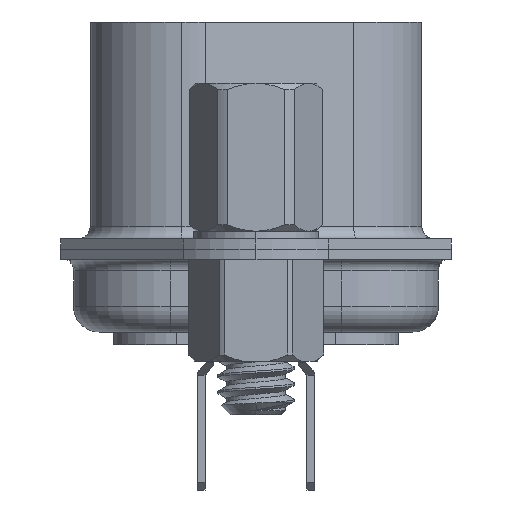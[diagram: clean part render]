
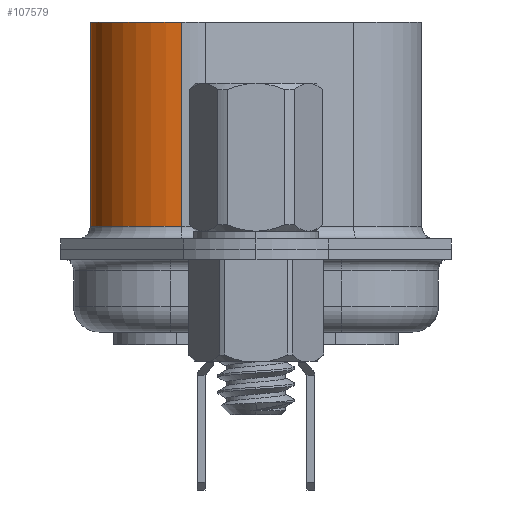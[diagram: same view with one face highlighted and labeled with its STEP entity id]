
A CAD part, left-side view. The second image highlights one B-rep face of the part: STEP entity #107579.
In plain terms, the highlighted cylindrical face has radius 3.6 mm (diameter 7.2 mm), a partial arc.
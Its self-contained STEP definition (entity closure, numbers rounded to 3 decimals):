
#177 = VECTOR ( 'NONE', #1300, 1000. ) ;
#1300 = DIRECTION ( 'NONE',  ( 0., 0., -1. ) ) ;
#10355 = AXIS2_PLACEMENT_3D ( 'NONE', #124263, #99683, #24302 ) ;
#10968 = AXIS2_PLACEMENT_3D ( 'NONE', #58347, #157442, #134458 ) ;
#18935 = EDGE_LOOP ( 'NONE', ( #150586, #107219, #74335, #55758 ) ) ;
#23056 = CARTESIAN_POINT ( 'NONE',  ( 4.79, 2.9, 1.3 ) ) ;
#24302 = DIRECTION ( 'NONE',  ( -1., 0., 0. ) ) ;
#31120 = DIRECTION ( 'NONE',  ( -1., 0., 0. ) ) ;
#37428 = CYLINDRICAL_SURFACE ( 'NONE', #10355, 3.6 ) ;
#48325 = CARTESIAN_POINT ( 'NONE',  ( 8.39, 6.5, 1.3 ) ) ;
#54092 = VERTEX_POINT ( 'NONE', #103294 ) ;
#55758 = ORIENTED_EDGE ( 'NONE', *, *, #150046, .T. ) ;
#55772 = VECTOR ( 'NONE', #66844, 1000. ) ;
#58289 = EDGE_CURVE ( 'NONE', #54092, #59859, #63576, .T. ) ;
#58347 = CARTESIAN_POINT ( 'NONE',  ( 8.39, 2.9, 9.3 ) ) ;
#59859 = VERTEX_POINT ( 'NONE', #23056 ) ;
#63576 = LINE ( 'NONE', #89766, #55772 ) ;
#66844 = DIRECTION ( 'NONE',  ( 0., 0., -1. ) ) ;
#66857 = LINE ( 'NONE', #89780, #177 ) ;
#68010 = CARTESIAN_POINT ( 'NONE',  ( 8.39, 2.9, 1.3 ) ) ;
#68803 = DIRECTION ( 'NONE',  ( 0., 0., 1. ) ) ;
#70940 = VERTEX_POINT ( 'NONE', #79677 ) ;
#71110 = CIRCLE ( 'NONE', #10968, 3.6 ) ;
#74335 = ORIENTED_EDGE ( 'NONE', *, *, #119852, .T. ) ;
#79677 = CARTESIAN_POINT ( 'NONE',  ( 8.39, 6.5, 9.3 ) ) ;
#89766 = CARTESIAN_POINT ( 'NONE',  ( 4.79, 2.9, 9.3 ) ) ;
#89780 = CARTESIAN_POINT ( 'NONE',  ( 8.39, 6.5, 9.3 ) ) ;
#99683 = DIRECTION ( 'NONE',  ( 0., 0., -1. ) ) ;
#103294 = CARTESIAN_POINT ( 'NONE',  ( 4.79, 2.9, 9.3 ) ) ;
#107219 = ORIENTED_EDGE ( 'NONE', *, *, #144455, .F. ) ;
#107579 = ADVANCED_FACE ( 'NONE', ( #147252 ), #37428, .T. ) ;
#108741 = AXIS2_PLACEMENT_3D ( 'NONE', #68010, #68803, #31120 ) ;
#119852 = EDGE_CURVE ( 'NONE', #70940, #121987, #66857, .T. ) ;
#121987 = VERTEX_POINT ( 'NONE', #48325 ) ;
#124263 = CARTESIAN_POINT ( 'NONE',  ( 8.39, 2.9, 9.3 ) ) ;
#134458 = DIRECTION ( 'NONE',  ( 1., 0., 0. ) ) ;
#142692 = CIRCLE ( 'NONE', #108741, 3.6 ) ;
#144455 = EDGE_CURVE ( 'NONE', #70940, #54092, #71110, .T. ) ;
#147252 = FACE_OUTER_BOUND ( 'NONE', #18935, .T. ) ;
#150046 = EDGE_CURVE ( 'NONE', #121987, #59859, #142692, .T. ) ;
#150586 = ORIENTED_EDGE ( 'NONE', *, *, #58289, .F. ) ;
#157442 = DIRECTION ( 'NONE',  ( 0., 0., 1. ) ) ;
